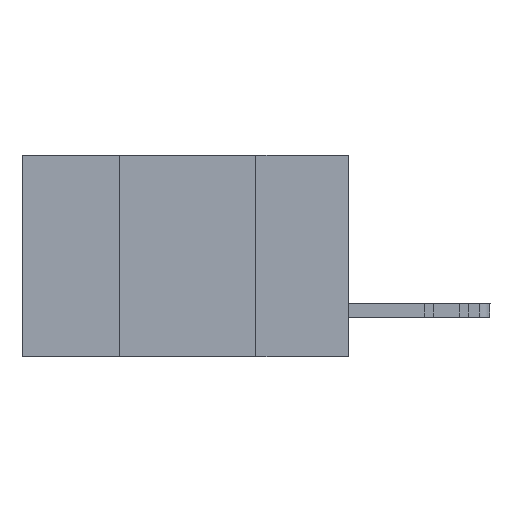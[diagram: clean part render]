
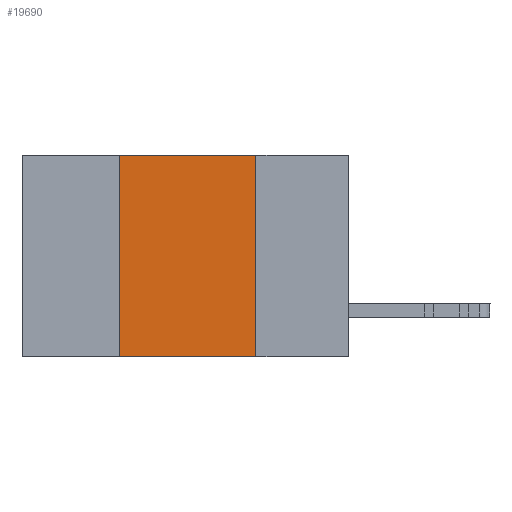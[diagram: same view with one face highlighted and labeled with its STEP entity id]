
A CAD part, left-side view. The second image highlights one B-rep face of the part: STEP entity #19690.
In plain terms, the highlighted planar face has unit normal (-1, 0, 0).
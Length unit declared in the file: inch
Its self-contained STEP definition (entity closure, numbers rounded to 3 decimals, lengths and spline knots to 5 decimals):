
#109 = ORIENTED_EDGE ( 'NONE', *, *, #16822, .T. ) ;
#1556 = DIRECTION ( 'NONE',  ( 0., 0., -1. ) ) ;
#1621 = ORIENTED_EDGE ( 'NONE', *, *, #6271, .F. ) ;
#2038 = CARTESIAN_POINT ( 'NONE',  ( 0., 0.42, -0.37 ) ) ;
#2208 = EDGE_CURVE ( 'NONE', #8784, #5824, #18179, .T. ) ;
#3219 = CARTESIAN_POINT ( 'NONE',  ( 0., 0.6, 0. ) ) ;
#3546 = EDGE_CURVE ( 'NONE', #13014, #8784, #16949, .T. ) ;
#4467 = CARTESIAN_POINT ( 'NONE',  ( 0., 0.17, -0.37 ) ) ;
#4585 = LINE ( 'NONE', #4467, #17397 ) ;
#4852 = VECTOR ( 'NONE', #5296, 39.37008 ) ;
#5296 = DIRECTION ( 'NONE',  ( 0., -1., 0. ) ) ;
#5824 = VERTEX_POINT ( 'NONE', #10136 ) ;
#6271 = EDGE_CURVE ( 'NONE', #5824, #20109, #4585, .T. ) ;
#7128 = CARTESIAN_POINT ( 'NONE',  ( 0., 0.42, -0.37 ) ) ;
#8324 = LINE ( 'NONE', #23044, #21427 ) ;
#8611 = CARTESIAN_POINT ( 'NONE',  ( 0., 0.17, -0.37 ) ) ;
#8784 = VERTEX_POINT ( 'NONE', #18461 ) ;
#8994 = PLANE ( 'NONE',  #9155 ) ;
#9155 = AXIS2_PLACEMENT_3D ( 'NONE', #3219, #18167, #1556 ) ;
#10136 = CARTESIAN_POINT ( 'NONE',  ( 0., 0.17, 0. ) ) ;
#13014 = VERTEX_POINT ( 'NONE', #7128 ) ;
#13858 = DIRECTION ( 'NONE',  ( 0., -1., 0. ) ) ;
#14667 = FACE_OUTER_BOUND ( 'NONE', #15588, .T. ) ;
#14790 = DIRECTION ( 'NONE',  ( 0., 0., 1. ) ) ;
#15588 = EDGE_LOOP ( 'NONE', ( #1621, #16933, #16412, #109 ) ) ;
#16412 = ORIENTED_EDGE ( 'NONE', *, *, #3546, .F. ) ;
#16822 = EDGE_CURVE ( 'NONE', #13014, #20109, #8324, .T. ) ;
#16933 = ORIENTED_EDGE ( 'NONE', *, *, #2208, .F. ) ;
#16949 = LINE ( 'NONE', #2038, #18297 ) ;
#17397 = VECTOR ( 'NONE', #18812, 39.37008 ) ;
#18167 = DIRECTION ( 'NONE',  ( 1., 0., 0. ) ) ;
#18179 = LINE ( 'NONE', #21809, #4852 ) ;
#18297 = VECTOR ( 'NONE', #14790, 39.37008 ) ;
#18461 = CARTESIAN_POINT ( 'NONE',  ( 0., 0.42, 0. ) ) ;
#18812 = DIRECTION ( 'NONE',  ( 0., 0., -1. ) ) ;
#19690 = ADVANCED_FACE ( 'NONE', ( #14667 ), #8994, .F. ) ;
#20109 = VERTEX_POINT ( 'NONE', #8611 ) ;
#21427 = VECTOR ( 'NONE', #13858, 39.37008 ) ;
#21809 = CARTESIAN_POINT ( 'NONE',  ( 0., 0.6, 0. ) ) ;
#23044 = CARTESIAN_POINT ( 'NONE',  ( 0., 0.6, -0.37 ) ) ;
